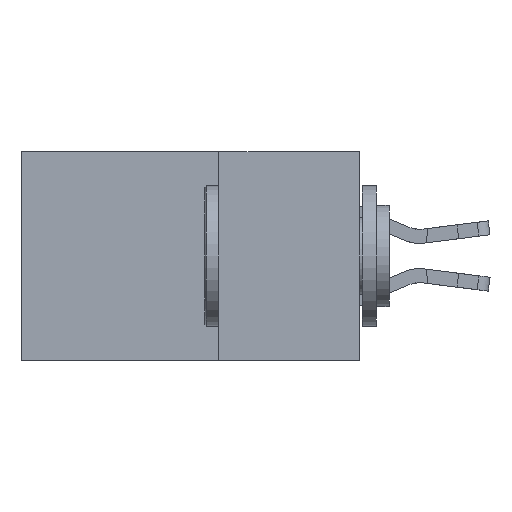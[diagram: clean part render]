
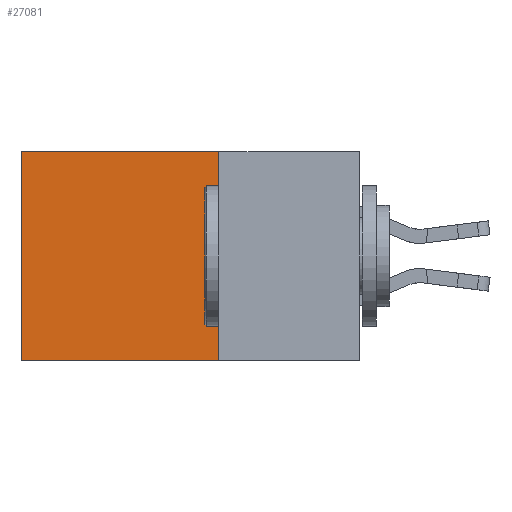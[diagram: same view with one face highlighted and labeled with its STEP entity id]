
A CAD part, left-side view. The second image highlights one B-rep face of the part: STEP entity #27081.
In plain terms, the highlighted planar face has unit normal (-1, 0, 0).
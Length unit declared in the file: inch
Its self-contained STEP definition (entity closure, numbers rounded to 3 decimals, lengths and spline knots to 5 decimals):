
#934 = CARTESIAN_POINT ( 'NONE',  ( 0.2875, 0.25, 0. ) ) ;
#1287 = VECTOR ( 'NONE', #25964, 39.37008 ) ;
#1491 = ORIENTED_EDGE ( 'NONE', *, *, #7211, .T. ) ;
#2065 = LINE ( 'NONE', #24705, #2769 ) ;
#2769 = VECTOR ( 'NONE', #13935, 39.37008 ) ;
#4235 = AXIS2_PLACEMENT_3D ( 'NONE', #25270, #12355, #27436 ) ;
#6306 = CARTESIAN_POINT ( 'NONE',  ( 0.2875, 0.6, -0.37 ) ) ;
#7211 = EDGE_CURVE ( 'NONE', #12102, #22768, #17967, .T. ) ;
#7264 = VECTOR ( 'NONE', #27953, 39.37008 ) ;
#7507 = CARTESIAN_POINT ( 'NONE',  ( 0.2875, 0.6, 0. ) ) ;
#8480 = FACE_OUTER_BOUND ( 'NONE', #18879, .T. ) ;
#8823 = VERTEX_POINT ( 'NONE', #25332 ) ;
#10304 = LINE ( 'NONE', #15033, #7264 ) ;
#12102 = VERTEX_POINT ( 'NONE', #7507 ) ;
#12115 = EDGE_CURVE ( 'NONE', #26017, #12102, #14724, .T. ) ;
#12355 = DIRECTION ( 'NONE',  ( 1., 0., 0. ) ) ;
#12779 = ORIENTED_EDGE ( 'NONE', *, *, #12115, .T. ) ;
#13069 = CARTESIAN_POINT ( 'NONE',  ( 0.2875, 0.6, 0. ) ) ;
#13280 = EDGE_CURVE ( 'NONE', #8823, #22768, #2065, .T. ) ;
#13935 = DIRECTION ( 'NONE',  ( 0., 1., 0. ) ) ;
#14055 = VECTOR ( 'NONE', #24768, 39.37008 ) ;
#14724 = LINE ( 'NONE', #934, #14055 ) ;
#15033 = CARTESIAN_POINT ( 'NONE',  ( 0.2875, 0.25, 0. ) ) ;
#17967 = LINE ( 'NONE', #13069, #1287 ) ;
#18115 = EDGE_CURVE ( 'NONE', #26017, #8823, #10304, .T. ) ;
#18752 = PLANE ( 'NONE',  #4235 ) ;
#18879 = EDGE_LOOP ( 'NONE', ( #1491, #21025, #22170, #12779 ) ) ;
#19798 = CARTESIAN_POINT ( 'NONE',  ( 0.2875, 0.25, 0. ) ) ;
#21025 = ORIENTED_EDGE ( 'NONE', *, *, #13280, .F. ) ;
#22170 = ORIENTED_EDGE ( 'NONE', *, *, #18115, .F. ) ;
#22768 = VERTEX_POINT ( 'NONE', #6306 ) ;
#24705 = CARTESIAN_POINT ( 'NONE',  ( 0.2875, 0.25, -0.37 ) ) ;
#24768 = DIRECTION ( 'NONE',  ( 0., 1., 0. ) ) ;
#25270 = CARTESIAN_POINT ( 'NONE',  ( 0.2875, 0.25, 0. ) ) ;
#25332 = CARTESIAN_POINT ( 'NONE',  ( 0.2875, 0.25, -0.37 ) ) ;
#25964 = DIRECTION ( 'NONE',  ( 0., 0., -1. ) ) ;
#26017 = VERTEX_POINT ( 'NONE', #19798 ) ;
#27081 = ADVANCED_FACE ( 'NONE', ( #8480 ), #18752, .F. ) ;
#27436 = DIRECTION ( 'NONE',  ( 0., 0., -1. ) ) ;
#27953 = DIRECTION ( 'NONE',  ( 0., 0., -1. ) ) ;
